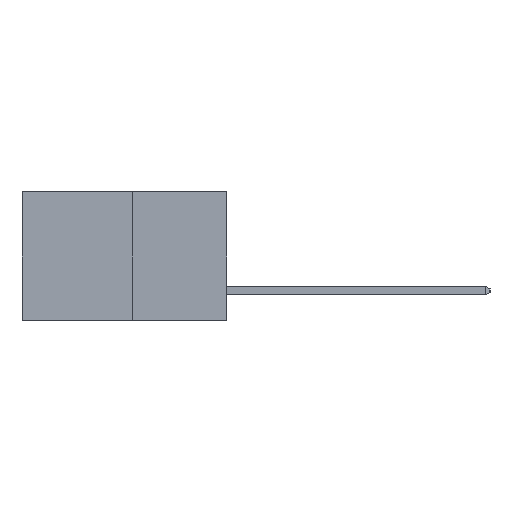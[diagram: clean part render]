
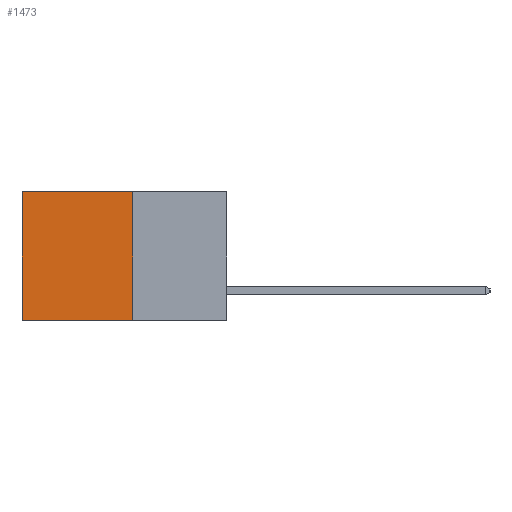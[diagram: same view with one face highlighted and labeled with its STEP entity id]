
A CAD part, left-side view. The second image highlights one B-rep face of the part: STEP entity #1473.
In plain terms, the highlighted planar face has unit normal (-1, 0, 0).
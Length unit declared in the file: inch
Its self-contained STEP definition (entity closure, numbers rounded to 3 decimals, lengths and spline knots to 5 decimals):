
#589 = LINE ( 'NONE', #9545, #2691 ) ;
#1280 = EDGE_CURVE ( 'NONE', #10103, #5075, #5068, .T. ) ;
#1463 = CARTESIAN_POINT ( 'NONE',  ( 0.277, 0.59, -0.37 ) ) ;
#1473 = ADVANCED_FACE ( 'NONE', ( #1780 ), #10401, .F. ) ;
#1551 = ORIENTED_EDGE ( 'NONE', *, *, #10660, .F. ) ;
#1780 = FACE_OUTER_BOUND ( 'NONE', #6303, .T. ) ;
#1886 = ORIENTED_EDGE ( 'NONE', *, *, #5840, .F. ) ;
#2691 = VECTOR ( 'NONE', #9492, 39.37008 ) ;
#3690 = VERTEX_POINT ( 'NONE', #6423 ) ;
#3713 = CARTESIAN_POINT ( 'NONE',  ( 0.277, 0.27, -0.37 ) ) ;
#3726 = CARTESIAN_POINT ( 'NONE',  ( 0.277, 0.59, 0. ) ) ;
#3758 = EDGE_CURVE ( 'NONE', #3690, #10103, #5921, .T. ) ;
#4594 = CARTESIAN_POINT ( 'NONE',  ( 0.277, 0.59, -0.37 ) ) ;
#4606 = DIRECTION ( 'NONE',  ( 0., 1., 0. ) ) ;
#5068 = LINE ( 'NONE', #1463, #7430 ) ;
#5075 = VERTEX_POINT ( 'NONE', #4594 ) ;
#5407 = CARTESIAN_POINT ( 'NONE',  ( 0.277, 0.27, -0.37 ) ) ;
#5472 = VECTOR ( 'NONE', #4606, 39.37008 ) ;
#5840 = EDGE_CURVE ( 'NONE', #3690, #6830, #589, .T. ) ;
#5921 = LINE ( 'NONE', #6006, #8256 ) ;
#5989 = ORIENTED_EDGE ( 'NONE', *, *, #3758, .T. ) ;
#6006 = CARTESIAN_POINT ( 'NONE',  ( 0.277, 0.27, 0. ) ) ;
#6134 = DIRECTION ( 'NONE',  ( 0., 1., 0. ) ) ;
#6303 = EDGE_LOOP ( 'NONE', ( #11052, #1551, #1886, #5989 ) ) ;
#6423 = CARTESIAN_POINT ( 'NONE',  ( 0.277, 0.27, 0. ) ) ;
#6642 = AXIS2_PLACEMENT_3D ( 'NONE', #10413, #10377, #10176 ) ;
#6830 = VERTEX_POINT ( 'NONE', #5407 ) ;
#7430 = VECTOR ( 'NONE', #9348, 39.37008 ) ;
#7532 = LINE ( 'NONE', #3713, #5472 ) ;
#8256 = VECTOR ( 'NONE', #6134, 39.37008 ) ;
#9348 = DIRECTION ( 'NONE',  ( 0., 0., -1. ) ) ;
#9492 = DIRECTION ( 'NONE',  ( 0., 0., -1. ) ) ;
#9545 = CARTESIAN_POINT ( 'NONE',  ( 0.277, 0.27, -0.37 ) ) ;
#10103 = VERTEX_POINT ( 'NONE', #3726 ) ;
#10176 = DIRECTION ( 'NONE',  ( 0., 0., -1. ) ) ;
#10377 = DIRECTION ( 'NONE',  ( 1., 0., 0. ) ) ;
#10401 = PLANE ( 'NONE',  #6642 ) ;
#10413 = CARTESIAN_POINT ( 'NONE',  ( 0.277, 0.27, -0.37 ) ) ;
#10660 = EDGE_CURVE ( 'NONE', #6830, #5075, #7532, .T. ) ;
#11052 = ORIENTED_EDGE ( 'NONE', *, *, #1280, .T. ) ;
